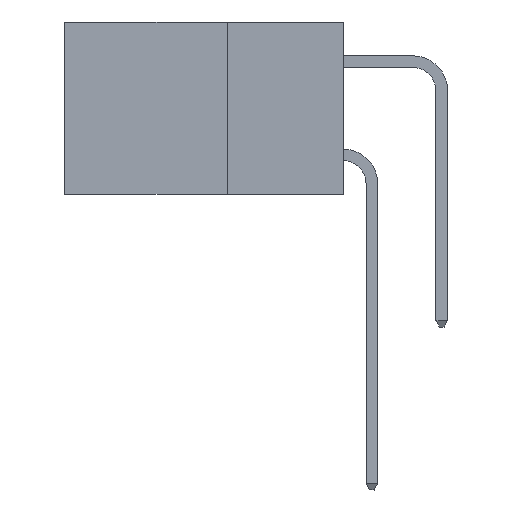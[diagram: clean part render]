
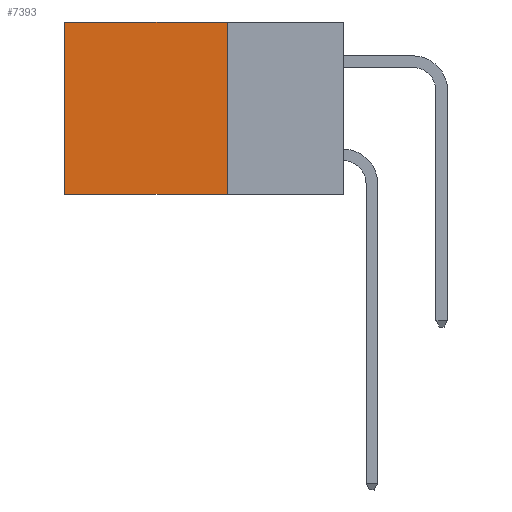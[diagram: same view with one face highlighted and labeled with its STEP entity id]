
A CAD part, left-side view. The second image highlights one B-rep face of the part: STEP entity #7393.
In plain terms, the highlighted planar face has unit normal (-1, 0, 0).
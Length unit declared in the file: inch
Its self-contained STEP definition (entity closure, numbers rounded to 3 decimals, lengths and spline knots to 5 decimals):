
#74 = DIRECTION ( 'NONE',  ( 0., 1., 0. ) ) ;
#1162 = VERTEX_POINT ( 'NONE', #7397 ) ;
#1814 = LINE ( 'NONE', #13477, #15589 ) ;
#2128 = DIRECTION ( 'NONE',  ( 1., 0., 0. ) ) ;
#2637 = CARTESIAN_POINT ( 'NONE',  ( 0.2615, 0.25, -0.37 ) ) ;
#3081 = VERTEX_POINT ( 'NONE', #18990 ) ;
#3271 = DIRECTION ( 'NONE',  ( 0., 0., -1. ) ) ;
#3570 = PLANE ( 'NONE',  #16370 ) ;
#3571 = EDGE_CURVE ( 'NONE', #10528, #1162, #7255, .T. ) ;
#4421 = CARTESIAN_POINT ( 'NONE',  ( 0.2615, 0.6, -0.37 ) ) ;
#6198 = ORIENTED_EDGE ( 'NONE', *, *, #13032, .T. ) ;
#7231 = VECTOR ( 'NONE', #3271, 39.37008 ) ;
#7255 = LINE ( 'NONE', #2637, #13987 ) ;
#7393 = ADVANCED_FACE ( 'NONE', ( #9355 ), #3570, .F. ) ;
#7397 = CARTESIAN_POINT ( 'NONE',  ( 0.2615, 0.25, -0.37 ) ) ;
#8002 = DIRECTION ( 'NONE',  ( 0., 0., -1. ) ) ;
#8041 = EDGE_CURVE ( 'NONE', #1162, #3081, #13085, .T. ) ;
#8976 = CARTESIAN_POINT ( 'NONE',  ( 0.2615, 0.6, 0. ) ) ;
#9033 = DIRECTION ( 'NONE',  ( 0., 1., 0. ) ) ;
#9355 = FACE_OUTER_BOUND ( 'NONE', #17339, .T. ) ;
#10480 = VERTEX_POINT ( 'NONE', #8976 ) ;
#10528 = VERTEX_POINT ( 'NONE', #10608 ) ;
#10580 = LINE ( 'NONE', #4421, #7231 ) ;
#10608 = CARTESIAN_POINT ( 'NONE',  ( 0.2615, 0.25, 0. ) ) ;
#11434 = ORIENTED_EDGE ( 'NONE', *, *, #12495, .T. ) ;
#12397 = ORIENTED_EDGE ( 'NONE', *, *, #8041, .F. ) ;
#12495 = EDGE_CURVE ( 'NONE', #10480, #3081, #10580, .T. ) ;
#13032 = EDGE_CURVE ( 'NONE', #10528, #10480, #1814, .T. ) ;
#13085 = LINE ( 'NONE', #13374, #18254 ) ;
#13374 = CARTESIAN_POINT ( 'NONE',  ( 0.2615, 0.25, -0.37 ) ) ;
#13477 = CARTESIAN_POINT ( 'NONE',  ( 0.2615, 0.25, 0. ) ) ;
#13976 = ORIENTED_EDGE ( 'NONE', *, *, #3571, .F. ) ;
#13987 = VECTOR ( 'NONE', #15939, 39.37008 ) ;
#15330 = CARTESIAN_POINT ( 'NONE',  ( 0.2615, 0.25, -0.37 ) ) ;
#15589 = VECTOR ( 'NONE', #9033, 39.37008 ) ;
#15939 = DIRECTION ( 'NONE',  ( 0., 0., -1. ) ) ;
#16370 = AXIS2_PLACEMENT_3D ( 'NONE', #15330, #2128, #8002 ) ;
#17339 = EDGE_LOOP ( 'NONE', ( #11434, #12397, #13976, #6198 ) ) ;
#18254 = VECTOR ( 'NONE', #74, 39.37008 ) ;
#18990 = CARTESIAN_POINT ( 'NONE',  ( 0.2615, 0.6, -0.37 ) ) ;
